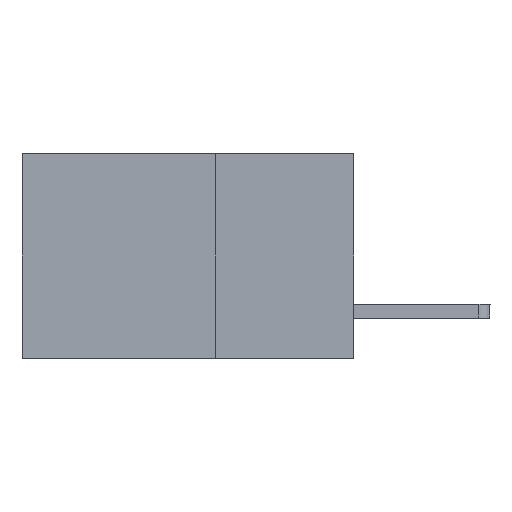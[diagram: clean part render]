
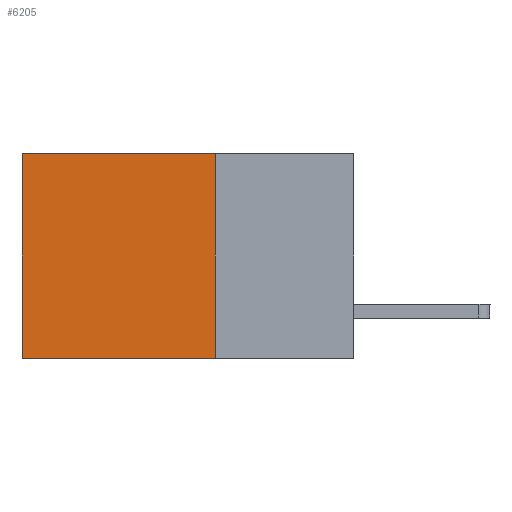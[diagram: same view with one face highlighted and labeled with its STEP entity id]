
A CAD part, left-side view. The second image highlights one B-rep face of the part: STEP entity #6205.
In plain terms, the highlighted planar face has unit normal (-1, 0, 0).
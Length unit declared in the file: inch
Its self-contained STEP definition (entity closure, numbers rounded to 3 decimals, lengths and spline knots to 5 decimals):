
#762 = LINE ( 'NONE', #5327, #6141 ) ;
#883 = EDGE_CURVE ( 'NONE', #1336, #7209, #5759, .T. ) ;
#1059 = DIRECTION ( 'NONE',  ( 0., 0., -1. ) ) ;
#1130 = DIRECTION ( 'NONE',  ( 0., 1., 0. ) ) ;
#1314 = ORIENTED_EDGE ( 'NONE', *, *, #883, .T. ) ;
#1336 = VERTEX_POINT ( 'NONE', #2913 ) ;
#1364 = DIRECTION ( 'NONE',  ( 1., 0., 0. ) ) ;
#2255 = ORIENTED_EDGE ( 'NONE', *, *, #3918, .F. ) ;
#2420 = EDGE_LOOP ( 'NONE', ( #1314, #4059, #2255, #3502 ) ) ;
#2815 = EDGE_CURVE ( 'NONE', #8409, #1336, #762, .T. ) ;
#2913 = CARTESIAN_POINT ( 'NONE',  ( 0.2875, 0.6, 0. ) ) ;
#3058 = VECTOR ( 'NONE', #10222, 39.37008 ) ;
#3502 = ORIENTED_EDGE ( 'NONE', *, *, #2815, .T. ) ;
#3918 = EDGE_CURVE ( 'NONE', #8409, #7857, #4878, .T. ) ;
#3938 = LINE ( 'NONE', #7754, #3058 ) ;
#4059 = ORIENTED_EDGE ( 'NONE', *, *, #6439, .F. ) ;
#4088 = CARTESIAN_POINT ( 'NONE',  ( 0.2875, 0.25, 0. ) ) ;
#4638 = VECTOR ( 'NONE', #5074, 39.37008 ) ;
#4878 = LINE ( 'NONE', #9224, #10219 ) ;
#5074 = DIRECTION ( 'NONE',  ( 0., 0., -1. ) ) ;
#5327 = CARTESIAN_POINT ( 'NONE',  ( 0.2875, 0.25, 0. ) ) ;
#5759 = LINE ( 'NONE', #6829, #4638 ) ;
#5845 = FACE_OUTER_BOUND ( 'NONE', #2420, .T. ) ;
#6141 = VECTOR ( 'NONE', #1130, 39.37008 ) ;
#6205 = ADVANCED_FACE ( 'NONE', ( #5845 ), #10080, .F. ) ;
#6216 = CARTESIAN_POINT ( 'NONE',  ( 0.2875, 0.6, -0.37 ) ) ;
#6439 = EDGE_CURVE ( 'NONE', #7857, #7209, #3938, .T. ) ;
#6829 = CARTESIAN_POINT ( 'NONE',  ( 0.2875, 0.6, 0. ) ) ;
#6890 = DIRECTION ( 'NONE',  ( 0., 0., -1. ) ) ;
#7006 = CARTESIAN_POINT ( 'NONE',  ( 0.2875, 0.25, 0. ) ) ;
#7209 = VERTEX_POINT ( 'NONE', #6216 ) ;
#7754 = CARTESIAN_POINT ( 'NONE',  ( 0.2875, 0.25, -0.37 ) ) ;
#7857 = VERTEX_POINT ( 'NONE', #10493 ) ;
#8409 = VERTEX_POINT ( 'NONE', #4088 ) ;
#8897 = AXIS2_PLACEMENT_3D ( 'NONE', #7006, #1364, #6890 ) ;
#9224 = CARTESIAN_POINT ( 'NONE',  ( 0.2875, 0.25, 0. ) ) ;
#10080 = PLANE ( 'NONE',  #8897 ) ;
#10219 = VECTOR ( 'NONE', #1059, 39.37008 ) ;
#10222 = DIRECTION ( 'NONE',  ( 0., 1., 0. ) ) ;
#10493 = CARTESIAN_POINT ( 'NONE',  ( 0.2875, 0.25, -0.37 ) ) ;
